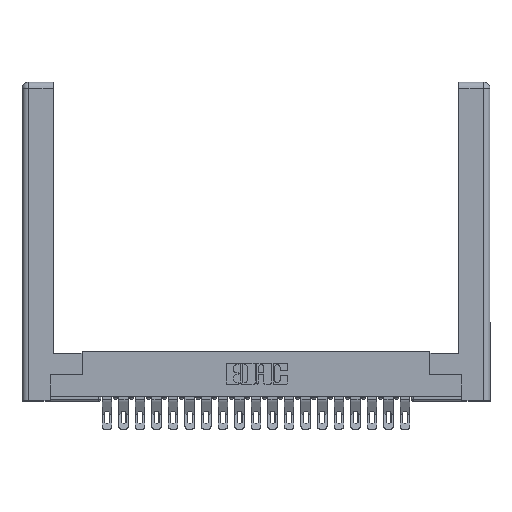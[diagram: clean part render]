
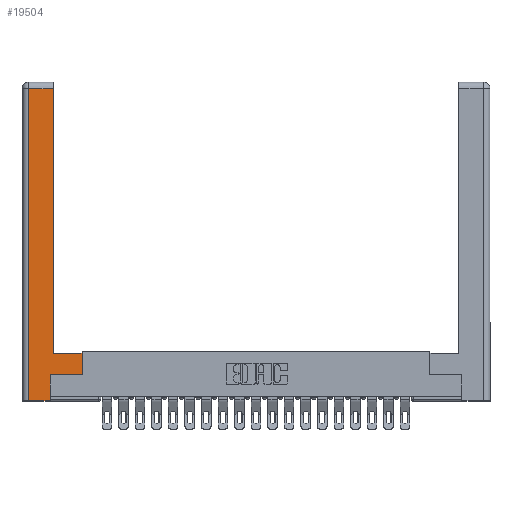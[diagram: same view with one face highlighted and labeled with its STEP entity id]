
A CAD part, top view. The second image highlights one B-rep face of the part: STEP entity #19504.
In plain terms, the highlighted planar face has unit normal (0, 0, 1).
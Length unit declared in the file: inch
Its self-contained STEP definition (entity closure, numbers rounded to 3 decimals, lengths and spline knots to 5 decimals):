
#44 = VERTEX_POINT ( 'NONE', #14706 ) ;
#1325 = DIRECTION ( 'NONE',  ( -1., 0., 0. ) ) ;
#1591 = DIRECTION ( 'NONE',  ( 1., 0., 0. ) ) ;
#1755 = CARTESIAN_POINT ( 'NONE',  ( 0.295, 3., 0. ) ) ;
#1826 = VECTOR ( 'NONE', #1591, 39.37008 ) ;
#1839 = DIRECTION ( 'NONE',  ( 0., 0., -1. ) ) ;
#2042 = VERTEX_POINT ( 'NONE', #17542 ) ;
#2479 = VERTEX_POINT ( 'NONE', #5421 ) ;
#2813 = DIRECTION ( 'NONE',  ( 0., 1., 0. ) ) ;
#3372 = VECTOR ( 'NONE', #22368, 39.37008 ) ;
#3525 = CARTESIAN_POINT ( 'NONE',  ( 0.295, 0.45, 0. ) ) ;
#3627 = ORIENTED_EDGE ( 'NONE', *, *, #15854, .T. ) ;
#3788 = LINE ( 'NONE', #19009, #7662 ) ;
#4271 = CARTESIAN_POINT ( 'NONE',  ( 0.295, 2.94, 0. ) ) ;
#4903 = AXIS2_PLACEMENT_3D ( 'NONE', #19217, #1839, #14131 ) ;
#5421 = CARTESIAN_POINT ( 'NONE',  ( 0.265, 0., 0. ) ) ;
#5491 = EDGE_CURVE ( 'NONE', #18140, #20513, #17171, .T. ) ;
#5634 = LINE ( 'NONE', #10291, #11708 ) ;
#5740 = ORIENTED_EDGE ( 'NONE', *, *, #22048, .T. ) ;
#5891 = EDGE_CURVE ( 'NONE', #10280, #2479, #12770, .T. ) ;
#6509 = LINE ( 'NONE', #19196, #1826 ) ;
#7135 = CARTESIAN_POINT ( 'NONE',  ( 0.265, 0.245, 0. ) ) ;
#7662 = VECTOR ( 'NONE', #17465, 39.37008 ) ;
#7790 = DIRECTION ( 'NONE',  ( -1., 0., 0. ) ) ;
#7811 = CARTESIAN_POINT ( 'NONE',  ( 0.0615, 2.94, 0. ) ) ;
#8652 = VECTOR ( 'NONE', #1325, 39.37008 ) ;
#8872 = EDGE_CURVE ( 'NONE', #2042, #10280, #5634, .T. ) ;
#9726 = EDGE_CURVE ( 'NONE', #20513, #2042, #11960, .T. ) ;
#10280 = VERTEX_POINT ( 'NONE', #21764 ) ;
#10291 = CARTESIAN_POINT ( 'NONE',  ( 0.0615, 0., 0. ) ) ;
#10642 = DIRECTION ( 'NONE',  ( 0., 1., 0. ) ) ;
#10909 = CARTESIAN_POINT ( 'NONE',  ( 0.265, 0.245, 0. ) ) ;
#11551 = ORIENTED_EDGE ( 'NONE', *, *, #5891, .T. ) ;
#11708 = VECTOR ( 'NONE', #20884, 39.37008 ) ;
#11960 = LINE ( 'NONE', #7811, #8652 ) ;
#12222 = VECTOR ( 'NONE', #10642, 39.37008 ) ;
#12770 = LINE ( 'NONE', #17218, #3372 ) ;
#12815 = LINE ( 'NONE', #10909, #18036 ) ;
#12956 = VERTEX_POINT ( 'NONE', #7135 ) ;
#13313 = CARTESIAN_POINT ( 'NONE',  ( 0.565, 0.245, 0. ) ) ;
#13495 = ORIENTED_EDGE ( 'NONE', *, *, #13630, .T. ) ;
#13630 = EDGE_CURVE ( 'NONE', #44, #18140, #21768, .T. ) ;
#13980 = PLANE ( 'NONE',  #4903 ) ;
#13985 = VERTEX_POINT ( 'NONE', #13313 ) ;
#14131 = DIRECTION ( 'NONE',  ( -1., 0., 0. ) ) ;
#14706 = CARTESIAN_POINT ( 'NONE',  ( 0.565, 0.45, 0. ) ) ;
#15854 = EDGE_CURVE ( 'NONE', #2479, #12956, #12815, .T. ) ;
#17171 = LINE ( 'NONE', #1755, #12222 ) ;
#17218 = CARTESIAN_POINT ( 'NONE',  ( 0.265, 0., 0. ) ) ;
#17465 = DIRECTION ( 'NONE',  ( 0., 1., 0. ) ) ;
#17542 = CARTESIAN_POINT ( 'NONE',  ( 0.0615, 2.94, 0. ) ) ;
#18036 = VECTOR ( 'NONE', #2813, 39.37008 ) ;
#18137 = VECTOR ( 'NONE', #7790, 39.37008 ) ;
#18140 = VERTEX_POINT ( 'NONE', #3525 ) ;
#18156 = ORIENTED_EDGE ( 'NONE', *, *, #8872, .T. ) ;
#18206 = CARTESIAN_POINT ( 'NONE',  ( 0.295, 0.45, 0. ) ) ;
#18468 = FACE_OUTER_BOUND ( 'NONE', #19797, .T. ) ;
#19009 = CARTESIAN_POINT ( 'NONE',  ( 0.565, 0.45, 0. ) ) ;
#19065 = ORIENTED_EDGE ( 'NONE', *, *, #5491, .T. ) ;
#19196 = CARTESIAN_POINT ( 'NONE',  ( 0.565, 0.245, 0. ) ) ;
#19217 = CARTESIAN_POINT ( 'NONE',  ( 0., 0., 0. ) ) ;
#19326 = ORIENTED_EDGE ( 'NONE', *, *, #9726, .T. ) ;
#19504 = ADVANCED_FACE ( 'NONE', ( #18468 ), #13980, .F. ) ;
#19797 = EDGE_LOOP ( 'NONE', ( #19065, #19326, #18156, #11551, #3627, #5740, #20834, #13495 ) ) ;
#20513 = VERTEX_POINT ( 'NONE', #4271 ) ;
#20564 = EDGE_CURVE ( 'NONE', #13985, #44, #3788, .T. ) ;
#20834 = ORIENTED_EDGE ( 'NONE', *, *, #20564, .T. ) ;
#20884 = DIRECTION ( 'NONE',  ( 0., -1., 0. ) ) ;
#21764 = CARTESIAN_POINT ( 'NONE',  ( 0.0615, 0., 0. ) ) ;
#21768 = LINE ( 'NONE', #18206, #18137 ) ;
#22048 = EDGE_CURVE ( 'NONE', #12956, #13985, #6509, .T. ) ;
#22368 = DIRECTION ( 'NONE',  ( 1., 0., 0. ) ) ;
